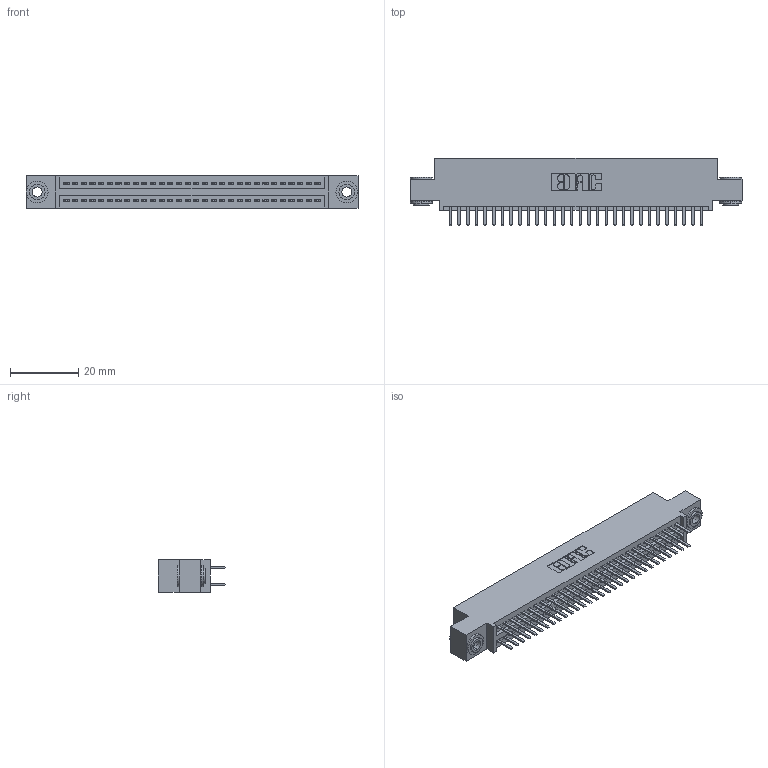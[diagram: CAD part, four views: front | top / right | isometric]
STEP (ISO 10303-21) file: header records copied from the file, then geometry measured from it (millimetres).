
FILE_DESCRIPTION (( 'STEP AP203' ), '1' );
FILE_NAME ('395-060-520-503.STEP', '2018-11-23T10:46:03', ( '' ), ( '' ), 'SwSTEP 2.0', 'SolidWorks 2016', '' );
FILE_SCHEMA (( 'CONFIG_CONTROL_DESIGN' ));
Length unit declared in the file: inch
Products named in the file (4): 345-292-001_345-293-120; 395-060-520-503; 345 Part_0.110 Offset - 0.156 Dia-TH; 345-250-002_345-250-002-102
Assembly tree (63 placements, depth 2):
  395-060-520-503
    345 Part_0.110 Offset - 0.156 Dia-TH
    345-292-001_345-293-120  x60
    345-250-002_345-250-002-102  x2
Bounding box: 97.41 x 19.68 x 9.4 mm (x, y, z)
Volume: 9270.7 mm3; surface area: 13712.8 mm2
Topology: 63 solids, 63 shells, 3408 faces, 9849 edges, 6402 vertices
Faces by surface type: plane 2194, cylinder 1206, cone 8
Entity records: 26050 total; most frequent: CARTESIAN_POINT 4367, ORIENTED_EDGE 4282, DIRECTION 3883, EDGE_CURVE 2141, VECTOR 1861, LINE 1861, VERTEX_POINT 1422, AXIS2_PLACEMENT_3D 1011
